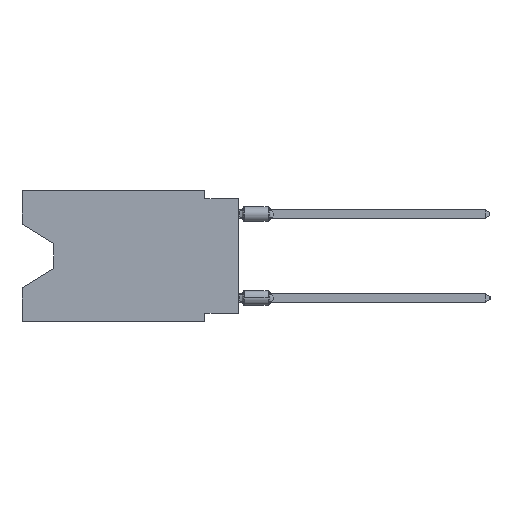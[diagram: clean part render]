
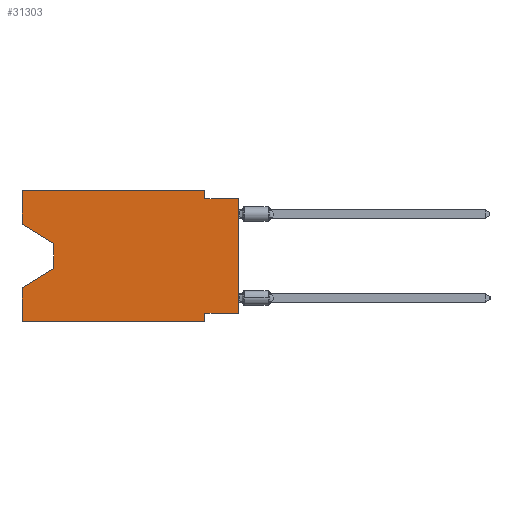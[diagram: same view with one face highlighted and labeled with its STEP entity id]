
A CAD part, left-side view. The second image highlights one B-rep face of the part: STEP entity #31303.
In plain terms, the highlighted planar face has unit normal (-1, 0, 0).
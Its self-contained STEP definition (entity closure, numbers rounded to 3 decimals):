
#72 = VECTOR ( 'NONE', #56554, 1000. ) ;
#139 = CARTESIAN_POINT ( 'NONE',  ( 0., 2.54, -9.906 ) ) ;
#639 = CARTESIAN_POINT ( 'NONE',  ( 0., 16.383, 0. ) ) ;
#921 = VECTOR ( 'NONE', #59464, 1000. ) ;
#947 = CARTESIAN_POINT ( 'NONE',  ( 0., 2.54, -0.635 ) ) ;
#1415 = CARTESIAN_POINT ( 'NONE',  ( 0., 16.383, 0. ) ) ;
#2954 = VECTOR ( 'NONE', #51920, 1000. ) ;
#3833 = CARTESIAN_POINT ( 'NONE',  ( 0., 0., -9.271 ) ) ;
#3873 = ORIENTED_EDGE ( 'NONE', *, *, #10305, .T. ) ;
#4790 = CARTESIAN_POINT ( 'NONE',  ( 0., 16.383, -9.906 ) ) ;
#5715 = CARTESIAN_POINT ( 'NONE',  ( 0., 16.383, 0. ) ) ;
#5809 = LINE ( 'NONE', #1415, #921 ) ;
#6248 = ORIENTED_EDGE ( 'NONE', *, *, #10465, .F. ) ;
#6997 = EDGE_CURVE ( 'NONE', #23911, #53280, #48373, .T. ) ;
#8171 = EDGE_CURVE ( 'NONE', #54029, #53461, #37421, .T. ) ;
#8364 = DIRECTION ( 'NONE',  ( 0., 0., -1. ) ) ;
#8434 = CARTESIAN_POINT ( 'NONE',  ( 0., 16.383, -7.36 ) ) ;
#9229 = CARTESIAN_POINT ( 'NONE',  ( 0., 2.54, -9.906 ) ) ;
#9548 = VERTEX_POINT ( 'NONE', #139 ) ;
#10305 = EDGE_CURVE ( 'NONE', #54566, #23911, #17544, .T. ) ;
#10452 = VECTOR ( 'NONE', #44589, 1000. ) ;
#10465 = EDGE_CURVE ( 'NONE', #26635, #23042, #5809, .T. ) ;
#11514 = CARTESIAN_POINT ( 'NONE',  ( 0., 2.54, 0. ) ) ;
#12059 = VERTEX_POINT ( 'NONE', #53219 ) ;
#12241 = CARTESIAN_POINT ( 'NONE',  ( 0., 0., -0.635 ) ) ;
#12554 = CARTESIAN_POINT ( 'NONE',  ( 0., 16.383, 0. ) ) ;
#12631 = ORIENTED_EDGE ( 'NONE', *, *, #23964, .T. ) ;
#12812 = EDGE_LOOP ( 'NONE', ( #3873, #32551, #12631, #6248, #47450, #52226, #14655, #25310, #31365, #18358, #19058, #36140 ) ) ;
#13073 = EDGE_CURVE ( 'NONE', #54029, #12059, #18414, .T. ) ;
#13100 = CARTESIAN_POINT ( 'NONE',  ( 0., 0., 0. ) ) ;
#14642 = DIRECTION ( 'NONE',  ( 0., -1., 0. ) ) ;
#14655 = ORIENTED_EDGE ( 'NONE', *, *, #8171, .F. ) ;
#16326 = LINE ( 'NONE', #53994, #10452 ) ;
#16479 = EDGE_CURVE ( 'NONE', #54566, #60386, #16326, .T. ) ;
#17544 = LINE ( 'NONE', #32596, #53011 ) ;
#17756 = VECTOR ( 'NONE', #32760, 1000. ) ;
#18358 = ORIENTED_EDGE ( 'NONE', *, *, #29962, .F. ) ;
#18414 = LINE ( 'NONE', #13100, #30212 ) ;
#19058 = ORIENTED_EDGE ( 'NONE', *, *, #28387, .F. ) ;
#19976 = VECTOR ( 'NONE', #23882, 1000. ) ;
#20159 = VECTOR ( 'NONE', #48980, 1000. ) ;
#20360 = VECTOR ( 'NONE', #45207, 1000. ) ;
#22197 = VERTEX_POINT ( 'NONE', #11514 ) ;
#22905 = VERTEX_POINT ( 'NONE', #947 ) ;
#23042 = VERTEX_POINT ( 'NONE', #8434 ) ;
#23339 = CARTESIAN_POINT ( 'NONE',  ( 0., 13.97, -4.013 ) ) ;
#23882 = DIRECTION ( 'NONE',  ( 0., 0., -1. ) ) ;
#23911 = VERTEX_POINT ( 'NONE', #23339 ) ;
#23964 = EDGE_CURVE ( 'NONE', #53280, #23042, #41880, .T. ) ;
#25310 = ORIENTED_EDGE ( 'NONE', *, *, #13073, .T. ) ;
#26635 = VERTEX_POINT ( 'NONE', #4790 ) ;
#27535 = DIRECTION ( 'NONE',  ( 0., 0., 1. ) ) ;
#28387 = EDGE_CURVE ( 'NONE', #60386, #22197, #44264, .T. ) ;
#28765 = CARTESIAN_POINT ( 'NONE',  ( 0., 16.383, -9.906 ) ) ;
#29085 = LINE ( 'NONE', #28765, #52461 ) ;
#29962 = EDGE_CURVE ( 'NONE', #22197, #22905, #61089, .T. ) ;
#30212 = VECTOR ( 'NONE', #27535, 1000. ) ;
#31303 = ADVANCED_FACE ( 'NONE', ( #41128 ), #52600, .F. ) ;
#31365 = ORIENTED_EDGE ( 'NONE', *, *, #53891, .F. ) ;
#31693 = DIRECTION ( 'NONE',  ( 0., 0., -1. ) ) ;
#32266 = AXIS2_PLACEMENT_3D ( 'NONE', #12554, #37873, #31693 ) ;
#32551 = ORIENTED_EDGE ( 'NONE', *, *, #6997, .T. ) ;
#32596 = CARTESIAN_POINT ( 'NONE',  ( 0., 16.383, -2.546 ) ) ;
#32760 = DIRECTION ( 'NONE',  ( 0., 0.855, -0.519 ) ) ;
#32980 = EDGE_CURVE ( 'NONE', #26635, #9548, #29085, .T. ) ;
#36140 = ORIENTED_EDGE ( 'NONE', *, *, #16479, .F. ) ;
#37421 = LINE ( 'NONE', #3833, #72 ) ;
#37873 = DIRECTION ( 'NONE',  ( 1., 0., 0. ) ) ;
#41128 = FACE_OUTER_BOUND ( 'NONE', #12812, .T. ) ;
#41880 = LINE ( 'NONE', #42191, #17756 ) ;
#42191 = CARTESIAN_POINT ( 'NONE',  ( 0., 13.97, -5.893 ) ) ;
#44264 = LINE ( 'NONE', #639, #20159 ) ;
#44589 = DIRECTION ( 'NONE',  ( 0., 0., 1. ) ) ;
#44664 = CARTESIAN_POINT ( 'NONE',  ( 0., 16.383, -2.546 ) ) ;
#45207 = DIRECTION ( 'NONE',  ( 0., -1., 0. ) ) ;
#47450 = ORIENTED_EDGE ( 'NONE', *, *, #32980, .T. ) ;
#48373 = LINE ( 'NONE', #48690, #19976 ) ;
#48690 = CARTESIAN_POINT ( 'NONE',  ( 0., 13.97, -4.013 ) ) ;
#48980 = DIRECTION ( 'NONE',  ( 0., -1., 0. ) ) ;
#49672 = EDGE_CURVE ( 'NONE', #53461, #9548, #61646, .T. ) ;
#51920 = DIRECTION ( 'NONE',  ( 0., 0., -1. ) ) ;
#52046 = DIRECTION ( 'NONE',  ( 0., -0.855, -0.519 ) ) ;
#52226 = ORIENTED_EDGE ( 'NONE', *, *, #49672, .F. ) ;
#52461 = VECTOR ( 'NONE', #14642, 1000. ) ;
#52600 = PLANE ( 'NONE',  #32266 ) ;
#53011 = VECTOR ( 'NONE', #52046, 1000. ) ;
#53219 = CARTESIAN_POINT ( 'NONE',  ( 0., 0., -0.635 ) ) ;
#53280 = VERTEX_POINT ( 'NONE', #61932 ) ;
#53461 = VERTEX_POINT ( 'NONE', #54678 ) ;
#53524 = CARTESIAN_POINT ( 'NONE',  ( 0., 0., -9.271 ) ) ;
#53891 = EDGE_CURVE ( 'NONE', #22905, #12059, #56996, .T. ) ;
#53994 = CARTESIAN_POINT ( 'NONE',  ( 0., 16.383, 0. ) ) ;
#54029 = VERTEX_POINT ( 'NONE', #53524 ) ;
#54566 = VERTEX_POINT ( 'NONE', #44664 ) ;
#54678 = CARTESIAN_POINT ( 'NONE',  ( 0., 2.54, -9.271 ) ) ;
#56554 = DIRECTION ( 'NONE',  ( 0., 1., 0. ) ) ;
#56996 = LINE ( 'NONE', #12241, #20360 ) ;
#59464 = DIRECTION ( 'NONE',  ( 0., 0., 1. ) ) ;
#60386 = VERTEX_POINT ( 'NONE', #5715 ) ;
#60413 = VECTOR ( 'NONE', #8364, 1000. ) ;
#61089 = LINE ( 'NONE', #62007, #60413 ) ;
#61646 = LINE ( 'NONE', #9229, #2954 ) ;
#61932 = CARTESIAN_POINT ( 'NONE',  ( 0., 13.97, -5.893 ) ) ;
#62007 = CARTESIAN_POINT ( 'NONE',  ( 0., 2.54, 0. ) ) ;
